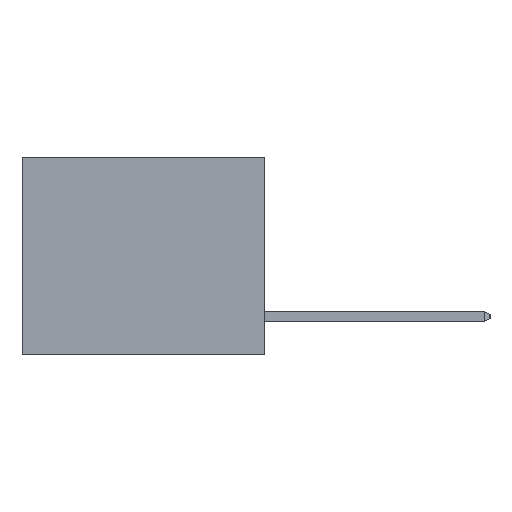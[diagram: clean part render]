
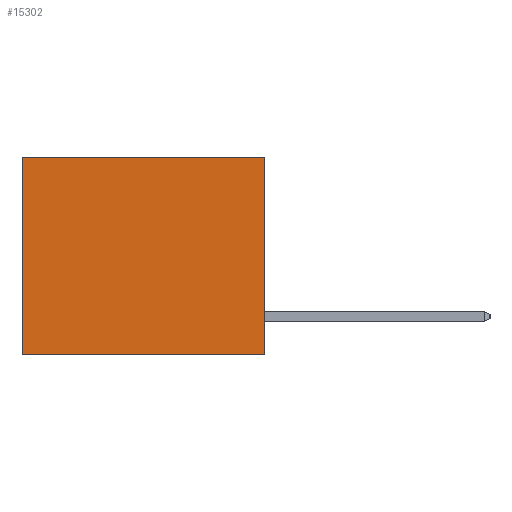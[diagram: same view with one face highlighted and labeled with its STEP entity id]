
A CAD part, left-side view. The second image highlights one B-rep face of the part: STEP entity #15302.
In plain terms, the highlighted planar face has unit normal (-1, 0, 0).
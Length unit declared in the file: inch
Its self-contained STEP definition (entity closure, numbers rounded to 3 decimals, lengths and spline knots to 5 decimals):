
#319 = LINE ( 'NONE', #9707, #599 ) ;
#599 = VECTOR ( 'NONE', #11971, 39.37008 ) ;
#882 = VERTEX_POINT ( 'NONE', #6012 ) ;
#1382 = EDGE_LOOP ( 'NONE', ( #7147, #12525, #1759, #18985 ) ) ;
#1759 = ORIENTED_EDGE ( 'NONE', *, *, #22726, .F. ) ;
#2919 = PLANE ( 'NONE',  #3606 ) ;
#3341 = CARTESIAN_POINT ( 'NONE',  ( 0.3165, 0., -0.49 ) ) ;
#3606 = AXIS2_PLACEMENT_3D ( 'NONE', #4523, #17159, #11614 ) ;
#4523 = CARTESIAN_POINT ( 'NONE',  ( 0.3165, 0., -0.49 ) ) ;
#5173 = DIRECTION ( 'NONE',  ( 0., 1., 0. ) ) ;
#6012 = CARTESIAN_POINT ( 'NONE',  ( 0.3165, 0., -0.49 ) ) ;
#7147 = ORIENTED_EDGE ( 'NONE', *, *, #15215, .T. ) ;
#9058 = LINE ( 'NONE', #9560, #19898 ) ;
#9560 = CARTESIAN_POINT ( 'NONE',  ( 0.3165, 0.6, -0.49 ) ) ;
#9707 = CARTESIAN_POINT ( 'NONE',  ( 0.3165, 0., -0.49 ) ) ;
#10712 = FACE_OUTER_BOUND ( 'NONE', #1382, .T. ) ;
#11614 = DIRECTION ( 'NONE',  ( 0., 0., -1. ) ) ;
#11971 = DIRECTION ( 'NONE',  ( 0., 0., -1. ) ) ;
#12525 = ORIENTED_EDGE ( 'NONE', *, *, #13395, .F. ) ;
#12985 = DIRECTION ( 'NONE',  ( 0., 0., -1. ) ) ;
#13395 = EDGE_CURVE ( 'NONE', #882, #22454, #16832, .T. ) ;
#15215 = EDGE_CURVE ( 'NONE', #18120, #22454, #9058, .T. ) ;
#15302 = ADVANCED_FACE ( 'NONE', ( #10712 ), #2919, .F. ) ;
#15736 = CARTESIAN_POINT ( 'NONE',  ( 0.3165, 0., 0. ) ) ;
#16531 = VECTOR ( 'NONE', #5173, 39.37008 ) ;
#16543 = CARTESIAN_POINT ( 'NONE',  ( 0.3165, 0.6, 0. ) ) ;
#16606 = CARTESIAN_POINT ( 'NONE',  ( 0.3165, 0., 0. ) ) ;
#16832 = LINE ( 'NONE', #3341, #16531 ) ;
#17159 = DIRECTION ( 'NONE',  ( 1., 0., 0. ) ) ;
#17745 = LINE ( 'NONE', #15736, #19427 ) ;
#18120 = VERTEX_POINT ( 'NONE', #16543 ) ;
#18539 = CARTESIAN_POINT ( 'NONE',  ( 0.3165, 0.6, -0.49 ) ) ;
#18985 = ORIENTED_EDGE ( 'NONE', *, *, #20151, .T. ) ;
#19427 = VECTOR ( 'NONE', #22952, 39.37008 ) ;
#19816 = VERTEX_POINT ( 'NONE', #16606 ) ;
#19898 = VECTOR ( 'NONE', #12985, 39.37008 ) ;
#20151 = EDGE_CURVE ( 'NONE', #19816, #18120, #17745, .T. ) ;
#22454 = VERTEX_POINT ( 'NONE', #18539 ) ;
#22726 = EDGE_CURVE ( 'NONE', #19816, #882, #319, .T. ) ;
#22952 = DIRECTION ( 'NONE',  ( 0., 1., 0. ) ) ;
